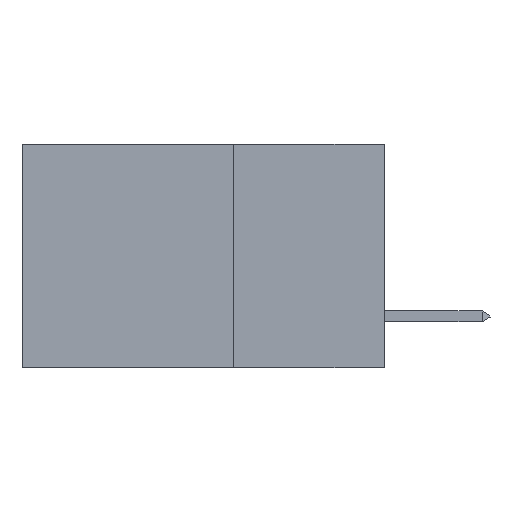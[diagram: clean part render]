
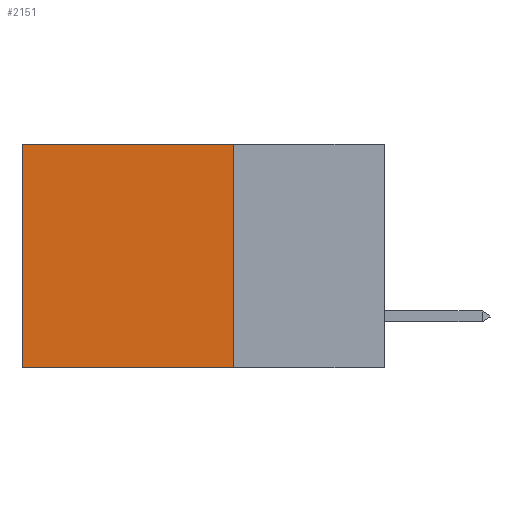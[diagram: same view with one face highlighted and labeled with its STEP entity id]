
A CAD part, left-side view. The second image highlights one B-rep face of the part: STEP entity #2151.
In plain terms, the highlighted planar face has unit normal (-1, 0, 0).
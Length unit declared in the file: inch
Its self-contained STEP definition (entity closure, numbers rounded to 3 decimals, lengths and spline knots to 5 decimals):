
#459 = DIRECTION ( 'NONE',  ( 0., 1., 0. ) ) ;
#578 = CARTESIAN_POINT ( 'NONE',  ( 0.2875, 0.6, 0. ) ) ;
#1683 = CARTESIAN_POINT ( 'NONE',  ( 0.2875, 0.25, -0.37 ) ) ;
#1829 = CARTESIAN_POINT ( 'NONE',  ( 0.2875, 0.6, -0.37 ) ) ;
#2078 = VECTOR ( 'NONE', #17716, 39.37008 ) ;
#2151 = ADVANCED_FACE ( 'NONE', ( #19518 ), #27011, .F. ) ;
#2764 = EDGE_LOOP ( 'NONE', ( #17321, #7515, #8579, #9124 ) ) ;
#2843 = CARTESIAN_POINT ( 'NONE',  ( 0.2875, 0.25, 0. ) ) ;
#2996 = LINE ( 'NONE', #1683, #28333 ) ;
#7515 = ORIENTED_EDGE ( 'NONE', *, *, #26218, .F. ) ;
#7952 = EDGE_CURVE ( 'NONE', #13902, #18282, #8127, .T. ) ;
#8127 = LINE ( 'NONE', #578, #2078 ) ;
#8418 = LINE ( 'NONE', #2843, #15306 ) ;
#8579 = ORIENTED_EDGE ( 'NONE', *, *, #24240, .F. ) ;
#9124 = ORIENTED_EDGE ( 'NONE', *, *, #9626, .T. ) ;
#9626 = EDGE_CURVE ( 'NONE', #15307, #13902, #8418, .T. ) ;
#11164 = DIRECTION ( 'NONE',  ( 0., 1., 0. ) ) ;
#12226 = CARTESIAN_POINT ( 'NONE',  ( 0.2875, 0.25, -0.37 ) ) ;
#13334 = CARTESIAN_POINT ( 'NONE',  ( 0.2875, 0.25, 0. ) ) ;
#13902 = VERTEX_POINT ( 'NONE', #17127 ) ;
#15306 = VECTOR ( 'NONE', #459, 39.37008 ) ;
#15307 = VERTEX_POINT ( 'NONE', #28768 ) ;
#17127 = CARTESIAN_POINT ( 'NONE',  ( 0.2875, 0.6, 0. ) ) ;
#17321 = ORIENTED_EDGE ( 'NONE', *, *, #7952, .T. ) ;
#17716 = DIRECTION ( 'NONE',  ( 0., 0., -1. ) ) ;
#18282 = VERTEX_POINT ( 'NONE', #1829 ) ;
#18637 = VECTOR ( 'NONE', #30384, 39.37008 ) ;
#19376 = DIRECTION ( 'NONE',  ( 0., 0., -1. ) ) ;
#19518 = FACE_OUTER_BOUND ( 'NONE', #2764, .T. ) ;
#19773 = DIRECTION ( 'NONE',  ( 1., 0., 0. ) ) ;
#24240 = EDGE_CURVE ( 'NONE', #15307, #25072, #25162, .T. ) ;
#25072 = VERTEX_POINT ( 'NONE', #12226 ) ;
#25162 = LINE ( 'NONE', #13334, #18637 ) ;
#26218 = EDGE_CURVE ( 'NONE', #25072, #18282, #2996, .T. ) ;
#26256 = AXIS2_PLACEMENT_3D ( 'NONE', #27118, #19773, #19376 ) ;
#27011 = PLANE ( 'NONE',  #26256 ) ;
#27118 = CARTESIAN_POINT ( 'NONE',  ( 0.2875, 0.25, 0. ) ) ;
#28333 = VECTOR ( 'NONE', #11164, 39.37008 ) ;
#28768 = CARTESIAN_POINT ( 'NONE',  ( 0.2875, 0.25, 0. ) ) ;
#30384 = DIRECTION ( 'NONE',  ( 0., 0., -1. ) ) ;
